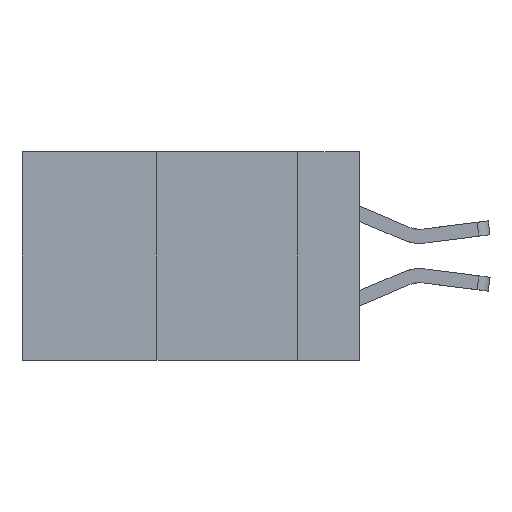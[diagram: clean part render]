
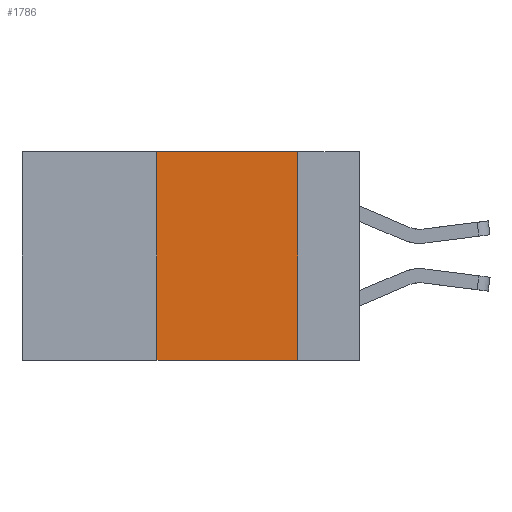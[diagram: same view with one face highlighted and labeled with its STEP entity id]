
A CAD part, left-side view. The second image highlights one B-rep face of the part: STEP entity #1786.
In plain terms, the highlighted planar face has unit normal (-1, 0, 0).
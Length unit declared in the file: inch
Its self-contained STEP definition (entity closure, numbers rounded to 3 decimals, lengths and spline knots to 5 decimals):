
#295 = LINE ( 'NONE', #2194, #4562 ) ;
#369 = EDGE_LOOP ( 'NONE', ( #433, #4635, #2258, #3511 ) ) ;
#433 = ORIENTED_EDGE ( 'NONE', *, *, #3223, .F. ) ;
#543 = DIRECTION ( 'NONE',  ( 1., 0., 0. ) ) ;
#893 = DIRECTION ( 'NONE',  ( 0., -1., 0. ) ) ;
#918 = VECTOR ( 'NONE', #893, 39.37008 ) ;
#1746 = AXIS2_PLACEMENT_3D ( 'NONE', #5498, #543, #6312 ) ;
#1786 = ADVANCED_FACE ( 'NONE', ( #9534 ), #2173, .F. ) ;
#2173 = PLANE ( 'NONE',  #1746 ) ;
#2194 = CARTESIAN_POINT ( 'NONE',  ( 0., 0.6, -0.37 ) ) ;
#2258 = ORIENTED_EDGE ( 'NONE', *, *, #9375, .F. ) ;
#2450 = EDGE_CURVE ( 'NONE', #5363, #4132, #5174, .T. ) ;
#3015 = LINE ( 'NONE', #5538, #3778 ) ;
#3094 = VECTOR ( 'NONE', #5819, 39.37008 ) ;
#3164 = DIRECTION ( 'NONE',  ( 0., 0., 1. ) ) ;
#3223 = EDGE_CURVE ( 'NONE', #4132, #9527, #4262, .T. ) ;
#3511 = ORIENTED_EDGE ( 'NONE', *, *, #6717, .T. ) ;
#3778 = VECTOR ( 'NONE', #3164, 39.37008 ) ;
#4095 = CARTESIAN_POINT ( 'NONE',  ( 0., 0.11, -0.37 ) ) ;
#4132 = VERTEX_POINT ( 'NONE', #6779 ) ;
#4262 = LINE ( 'NONE', #8334, #3094 ) ;
#4562 = VECTOR ( 'NONE', #9580, 39.37008 ) ;
#4635 = ORIENTED_EDGE ( 'NONE', *, *, #2450, .F. ) ;
#5174 = LINE ( 'NONE', #9913, #918 ) ;
#5360 = CARTESIAN_POINT ( 'NONE',  ( 0., 0.36, -0.37 ) ) ;
#5363 = VERTEX_POINT ( 'NONE', #6832 ) ;
#5498 = CARTESIAN_POINT ( 'NONE',  ( 0., 0.6, 0. ) ) ;
#5538 = CARTESIAN_POINT ( 'NONE',  ( 0., 0.36, 0. ) ) ;
#5819 = DIRECTION ( 'NONE',  ( 0., 0., -1. ) ) ;
#6312 = DIRECTION ( 'NONE',  ( 0., 0., -1. ) ) ;
#6717 = EDGE_CURVE ( 'NONE', #8117, #9527, #295, .T. ) ;
#6779 = CARTESIAN_POINT ( 'NONE',  ( 0., 0.11, 0. ) ) ;
#6832 = CARTESIAN_POINT ( 'NONE',  ( 0., 0.36, 0. ) ) ;
#8117 = VERTEX_POINT ( 'NONE', #5360 ) ;
#8334 = CARTESIAN_POINT ( 'NONE',  ( 0., 0.11, 0. ) ) ;
#9375 = EDGE_CURVE ( 'NONE', #8117, #5363, #3015, .T. ) ;
#9527 = VERTEX_POINT ( 'NONE', #4095 ) ;
#9534 = FACE_OUTER_BOUND ( 'NONE', #369, .T. ) ;
#9580 = DIRECTION ( 'NONE',  ( 0., -1., 0. ) ) ;
#9913 = CARTESIAN_POINT ( 'NONE',  ( 0., 0.6, 0. ) ) ;
